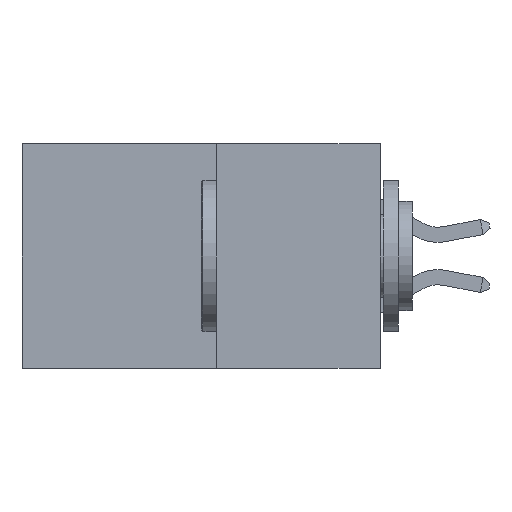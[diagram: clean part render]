
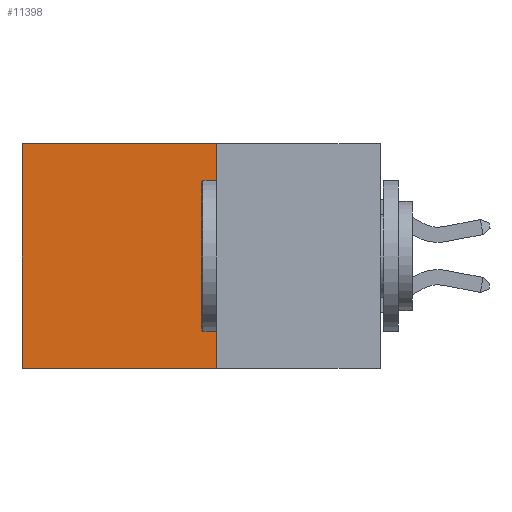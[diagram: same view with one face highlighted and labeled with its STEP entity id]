
A CAD part, left-side view. The second image highlights one B-rep face of the part: STEP entity #11398.
In plain terms, the highlighted planar face has unit normal (-1, 0, 0).
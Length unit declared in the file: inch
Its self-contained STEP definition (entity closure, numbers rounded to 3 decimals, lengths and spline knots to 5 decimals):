
#1945 = EDGE_LOOP ( 'NONE', ( #4939, #24948, #10311, #8501 ) ) ;
#2717 = CARTESIAN_POINT ( 'NONE',  ( 0.277, 0.27, -0.37 ) ) ;
#2921 = DIRECTION ( 'NONE',  ( 0., 0., -1. ) ) ;
#2978 = LINE ( 'NONE', #18383, #25925 ) ;
#4939 = ORIENTED_EDGE ( 'NONE', *, *, #13743, .T. ) ;
#6543 = CARTESIAN_POINT ( 'NONE',  ( 0.277, 0.59, -0.37 ) ) ;
#7053 = CARTESIAN_POINT ( 'NONE',  ( 0.277, 0.27, -0.37 ) ) ;
#8103 = VECTOR ( 'NONE', #8801, 39.37008 ) ;
#8168 = VECTOR ( 'NONE', #25997, 39.37008 ) ;
#8501 = ORIENTED_EDGE ( 'NONE', *, *, #13492, .T. ) ;
#8774 = LINE ( 'NONE', #26582, #8103 ) ;
#8801 = DIRECTION ( 'NONE',  ( 0., 1., 0. ) ) ;
#9041 = EDGE_CURVE ( 'NONE', #9911, #16924, #2978, .T. ) ;
#9244 = DIRECTION ( 'NONE',  ( 0., 0., -1. ) ) ;
#9911 = VERTEX_POINT ( 'NONE', #24564 ) ;
#10261 = LINE ( 'NONE', #23775, #8168 ) ;
#10311 = ORIENTED_EDGE ( 'NONE', *, *, #9041, .F. ) ;
#11368 = AXIS2_PLACEMENT_3D ( 'NONE', #7053, #22537, #9244 ) ;
#11398 = ADVANCED_FACE ( 'NONE', ( #27734 ), #15875, .F. ) ;
#12739 = VERTEX_POINT ( 'NONE', #6543 ) ;
#12954 = LINE ( 'NONE', #16788, #24055 ) ;
#13492 = EDGE_CURVE ( 'NONE', #9911, #14473, #8774, .T. ) ;
#13743 = EDGE_CURVE ( 'NONE', #14473, #12739, #12954, .T. ) ;
#14473 = VERTEX_POINT ( 'NONE', #25755 ) ;
#15875 = PLANE ( 'NONE',  #11368 ) ;
#16788 = CARTESIAN_POINT ( 'NONE',  ( 0.277, 0.59, -0.37 ) ) ;
#16924 = VERTEX_POINT ( 'NONE', #2717 ) ;
#18383 = CARTESIAN_POINT ( 'NONE',  ( 0.277, 0.27, -0.37 ) ) ;
#18996 = DIRECTION ( 'NONE',  ( 0., 0., -1. ) ) ;
#22537 = DIRECTION ( 'NONE',  ( 1., 0., 0. ) ) ;
#23775 = CARTESIAN_POINT ( 'NONE',  ( 0.277, 0.27, -0.37 ) ) ;
#24055 = VECTOR ( 'NONE', #18996, 39.37008 ) ;
#24148 = EDGE_CURVE ( 'NONE', #16924, #12739, #10261, .T. ) ;
#24564 = CARTESIAN_POINT ( 'NONE',  ( 0.277, 0.27, 0. ) ) ;
#24948 = ORIENTED_EDGE ( 'NONE', *, *, #24148, .F. ) ;
#25755 = CARTESIAN_POINT ( 'NONE',  ( 0.277, 0.59, 0. ) ) ;
#25925 = VECTOR ( 'NONE', #2921, 39.37008 ) ;
#25997 = DIRECTION ( 'NONE',  ( 0., 1., 0. ) ) ;
#26582 = CARTESIAN_POINT ( 'NONE',  ( 0.277, 0.27, 0. ) ) ;
#27734 = FACE_OUTER_BOUND ( 'NONE', #1945, .T. ) ;
